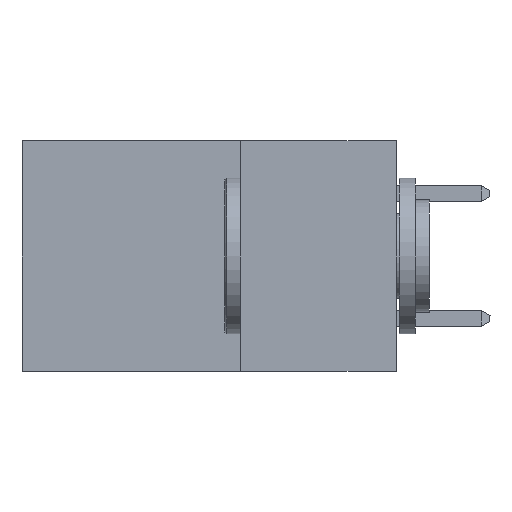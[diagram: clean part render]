
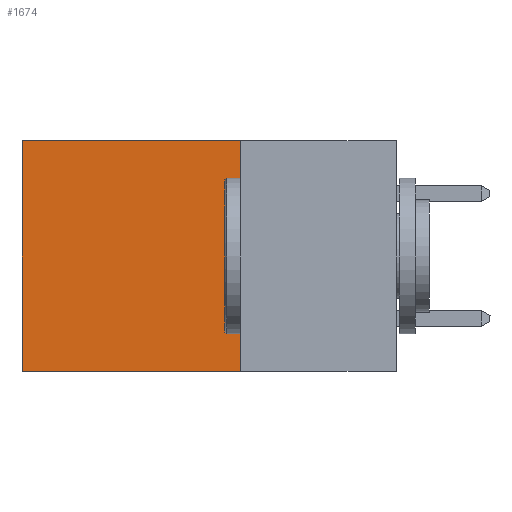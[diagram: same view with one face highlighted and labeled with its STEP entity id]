
A CAD part, left-side view. The second image highlights one B-rep face of the part: STEP entity #1674.
In plain terms, the highlighted planar face has unit normal (-1, 0, 0).
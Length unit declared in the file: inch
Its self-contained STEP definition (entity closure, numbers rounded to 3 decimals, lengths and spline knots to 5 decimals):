
#30 = ORIENTED_EDGE ( 'NONE', *, *, #5603, .F. ) ;
#139 = ORIENTED_EDGE ( 'NONE', *, *, #2263, .F. ) ;
#228 = VERTEX_POINT ( 'NONE', #9151 ) ;
#385 = ORIENTED_EDGE ( 'NONE', *, *, #2075, .T. ) ;
#481 = FACE_OUTER_BOUND ( 'NONE', #7211, .T. ) ;
#1225 = CARTESIAN_POINT ( 'NONE',  ( 0.2615, 0.25, 0. ) ) ;
#1231 = VERTEX_POINT ( 'NONE', #8653 ) ;
#1548 = AXIS2_PLACEMENT_3D ( 'NONE', #3564, #2349, #8716 ) ;
#1619 = EDGE_CURVE ( 'NONE', #1231, #3238, #5075, .T. ) ;
#1674 = ADVANCED_FACE ( 'NONE', ( #481 ), #7032, .F. ) ;
#2062 = ORIENTED_EDGE ( 'NONE', *, *, #1619, .T. ) ;
#2075 = EDGE_CURVE ( 'NONE', #7071, #1231, #3156, .T. ) ;
#2259 = VECTOR ( 'NONE', #8915, 39.37008 ) ;
#2263 = EDGE_CURVE ( 'NONE', #228, #3238, #6483, .T. ) ;
#2349 = DIRECTION ( 'NONE',  ( 1., 0., 0. ) ) ;
#2509 = LINE ( 'NONE', #4147, #2259 ) ;
#3156 = LINE ( 'NONE', #8948, #6593 ) ;
#3238 = VERTEX_POINT ( 'NONE', #5185 ) ;
#3564 = CARTESIAN_POINT ( 'NONE',  ( 0.2615, 0.25, -0.37 ) ) ;
#4147 = CARTESIAN_POINT ( 'NONE',  ( 0.2615, 0.25, -0.37 ) ) ;
#5075 = LINE ( 'NONE', #7920, #6910 ) ;
#5185 = CARTESIAN_POINT ( 'NONE',  ( 0.2615, 0.6, -0.37 ) ) ;
#5603 = EDGE_CURVE ( 'NONE', #7071, #228, #2509, .T. ) ;
#5639 = DIRECTION ( 'NONE',  ( 0., 0., -1. ) ) ;
#6483 = LINE ( 'NONE', #7126, #7844 ) ;
#6593 = VECTOR ( 'NONE', #9000, 39.37008 ) ;
#6910 = VECTOR ( 'NONE', #5639, 39.37008 ) ;
#7032 = PLANE ( 'NONE',  #1548 ) ;
#7071 = VERTEX_POINT ( 'NONE', #1225 ) ;
#7117 = DIRECTION ( 'NONE',  ( 0., 1., 0. ) ) ;
#7126 = CARTESIAN_POINT ( 'NONE',  ( 0.2615, 0.25, -0.37 ) ) ;
#7211 = EDGE_LOOP ( 'NONE', ( #2062, #139, #30, #385 ) ) ;
#7844 = VECTOR ( 'NONE', #7117, 39.37008 ) ;
#7920 = CARTESIAN_POINT ( 'NONE',  ( 0.2615, 0.6, -0.37 ) ) ;
#8653 = CARTESIAN_POINT ( 'NONE',  ( 0.2615, 0.6, 0. ) ) ;
#8716 = DIRECTION ( 'NONE',  ( 0., 0., -1. ) ) ;
#8915 = DIRECTION ( 'NONE',  ( 0., 0., -1. ) ) ;
#8948 = CARTESIAN_POINT ( 'NONE',  ( 0.2615, 0.25, 0. ) ) ;
#9000 = DIRECTION ( 'NONE',  ( 0., 1., 0. ) ) ;
#9151 = CARTESIAN_POINT ( 'NONE',  ( 0.2615, 0.25, -0.37 ) ) ;
